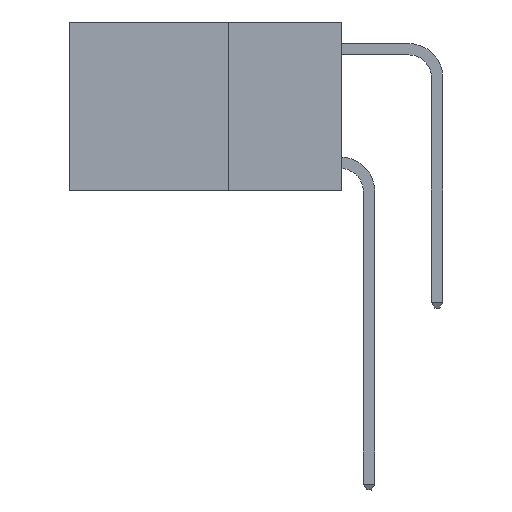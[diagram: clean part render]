
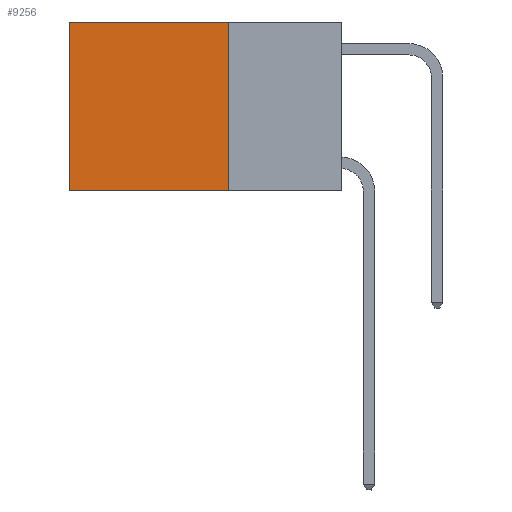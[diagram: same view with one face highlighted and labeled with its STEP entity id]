
A CAD part, left-side view. The second image highlights one B-rep face of the part: STEP entity #9256.
In plain terms, the highlighted planar face has unit normal (-1, 0, 0).
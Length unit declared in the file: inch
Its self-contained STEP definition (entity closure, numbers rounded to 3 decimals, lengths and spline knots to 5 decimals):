
#457 = VERTEX_POINT ( 'NONE', #3893 ) ;
#828 = EDGE_CURVE ( 'NONE', #5611, #4173, #8993, .T. ) ;
#902 = EDGE_LOOP ( 'NONE', ( #3475, #13205, #13065, #15405 ) ) ;
#1221 = EDGE_CURVE ( 'NONE', #4173, #457, #9840, .T. ) ;
#2235 = DIRECTION ( 'NONE',  ( 0., 0., -1. ) ) ;
#3475 = ORIENTED_EDGE ( 'NONE', *, *, #10244, .T. ) ;
#3893 = CARTESIAN_POINT ( 'NONE',  ( 0.2625, 0.6, -0.37 ) ) ;
#4173 = VERTEX_POINT ( 'NONE', #7399 ) ;
#4696 = CARTESIAN_POINT ( 'NONE',  ( 0.2625, 0.6, 0. ) ) ;
#5124 = DIRECTION ( 'NONE',  ( 0., 1., 0. ) ) ;
#5611 = VERTEX_POINT ( 'NONE', #12396 ) ;
#6137 = DIRECTION ( 'NONE',  ( 0., 0., -1. ) ) ;
#7399 = CARTESIAN_POINT ( 'NONE',  ( 0.2625, 0.25, -0.37 ) ) ;
#7450 = VECTOR ( 'NONE', #2235, 39.37008 ) ;
#7803 = VECTOR ( 'NONE', #16762, 39.37008 ) ;
#7987 = CARTESIAN_POINT ( 'NONE',  ( 0.2625, 0.25, 0. ) ) ;
#8993 = LINE ( 'NONE', #11008, #15538 ) ;
#9256 = ADVANCED_FACE ( 'NONE', ( #16514 ), #15848, .F. ) ;
#9361 = DIRECTION ( 'NONE',  ( 0., 0., -1. ) ) ;
#9717 = AXIS2_PLACEMENT_3D ( 'NONE', #7987, #17111, #9361 ) ;
#9840 = LINE ( 'NONE', #13716, #12926 ) ;
#10244 = EDGE_CURVE ( 'NONE', #13000, #457, #14483, .T. ) ;
#10337 = CARTESIAN_POINT ( 'NONE',  ( 0.2625, 0.25, 0. ) ) ;
#11008 = CARTESIAN_POINT ( 'NONE',  ( 0.2625, 0.25, 0. ) ) ;
#12396 = CARTESIAN_POINT ( 'NONE',  ( 0.2625, 0.25, 0. ) ) ;
#12926 = VECTOR ( 'NONE', #5124, 39.37008 ) ;
#13000 = VERTEX_POINT ( 'NONE', #4696 ) ;
#13065 = ORIENTED_EDGE ( 'NONE', *, *, #828, .F. ) ;
#13205 = ORIENTED_EDGE ( 'NONE', *, *, #1221, .F. ) ;
#13716 = CARTESIAN_POINT ( 'NONE',  ( 0.2625, 0.25, -0.37 ) ) ;
#14190 = CARTESIAN_POINT ( 'NONE',  ( 0.2625, 0.6, 0. ) ) ;
#14403 = LINE ( 'NONE', #10337, #7803 ) ;
#14483 = LINE ( 'NONE', #14190, #7450 ) ;
#15405 = ORIENTED_EDGE ( 'NONE', *, *, #15504, .T. ) ;
#15504 = EDGE_CURVE ( 'NONE', #5611, #13000, #14403, .T. ) ;
#15538 = VECTOR ( 'NONE', #6137, 39.37008 ) ;
#15848 = PLANE ( 'NONE',  #9717 ) ;
#16514 = FACE_OUTER_BOUND ( 'NONE', #902, .T. ) ;
#16762 = DIRECTION ( 'NONE',  ( 0., 1., 0. ) ) ;
#17111 = DIRECTION ( 'NONE',  ( 1., 0., 0. ) ) ;
